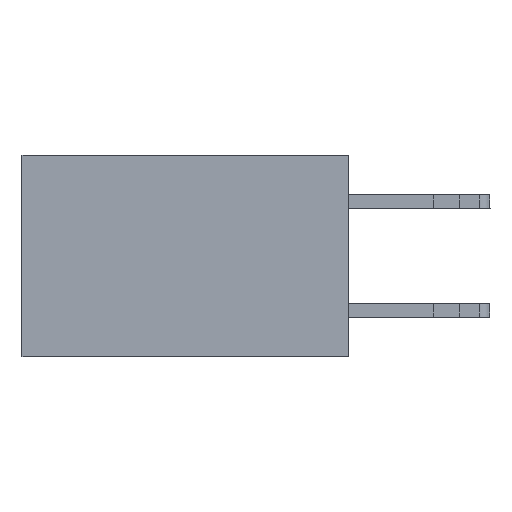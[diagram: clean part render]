
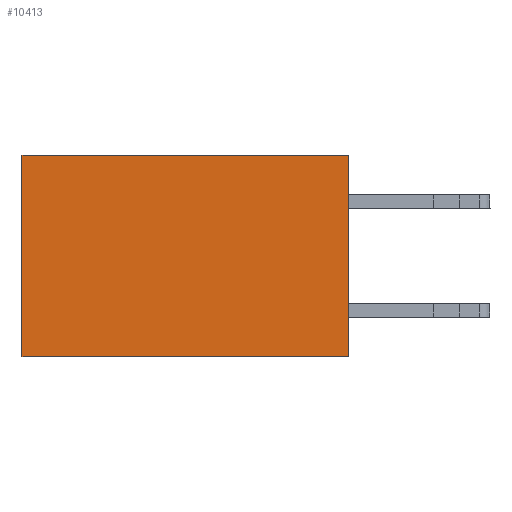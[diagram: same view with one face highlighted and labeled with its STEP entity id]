
A CAD part, left-side view. The second image highlights one B-rep face of the part: STEP entity #10413.
In plain terms, the highlighted planar face has unit normal (-1, 0, 0).
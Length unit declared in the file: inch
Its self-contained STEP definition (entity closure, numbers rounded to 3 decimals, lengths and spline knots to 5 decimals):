
#1106 = CARTESIAN_POINT ( 'NONE',  ( 0.2615, 0., -0.37 ) ) ;
#1721 = EDGE_CURVE ( 'NONE', #8797, #2682, #7178, .T. ) ;
#1941 = DIRECTION ( 'NONE',  ( 0., 0., -1. ) ) ;
#2469 = VECTOR ( 'NONE', #15292, 39.37008 ) ;
#2682 = VERTEX_POINT ( 'NONE', #7598 ) ;
#3089 = EDGE_CURVE ( 'NONE', #3127, #8797, #10516, .T. ) ;
#3127 = VERTEX_POINT ( 'NONE', #13555 ) ;
#3202 = ORIENTED_EDGE ( 'NONE', *, *, #16057, .T. ) ;
#3673 = DIRECTION ( 'NONE',  ( 1., 0., 0. ) ) ;
#4519 = AXIS2_PLACEMENT_3D ( 'NONE', #15950, #3673, #1941 ) ;
#4610 = ORIENTED_EDGE ( 'NONE', *, *, #1721, .F. ) ;
#5756 = DIRECTION ( 'NONE',  ( 0., 1., 0. ) ) ;
#5935 = CARTESIAN_POINT ( 'NONE',  ( 0.2615, 0.6, 0. ) ) ;
#7178 = LINE ( 'NONE', #11849, #13612 ) ;
#7293 = LINE ( 'NONE', #16848, #8883 ) ;
#7337 = DIRECTION ( 'NONE',  ( 0., 0., -1. ) ) ;
#7400 = ORIENTED_EDGE ( 'NONE', *, *, #3089, .F. ) ;
#7489 = DIRECTION ( 'NONE',  ( 0., 1., 0. ) ) ;
#7598 = CARTESIAN_POINT ( 'NONE',  ( 0.2615, 0.6, -0.37 ) ) ;
#7959 = EDGE_CURVE ( 'NONE', #9068, #2682, #10483, .T. ) ;
#8302 = ORIENTED_EDGE ( 'NONE', *, *, #7959, .T. ) ;
#8429 = PLANE ( 'NONE',  #4519 ) ;
#8797 = VERTEX_POINT ( 'NONE', #19574 ) ;
#8883 = VECTOR ( 'NONE', #7489, 39.37008 ) ;
#9068 = VERTEX_POINT ( 'NONE', #5935 ) ;
#10413 = ADVANCED_FACE ( 'NONE', ( #12794 ), #8429, .F. ) ;
#10483 = LINE ( 'NONE', #16701, #17143 ) ;
#10516 = LINE ( 'NONE', #1106, #2469 ) ;
#11034 = EDGE_LOOP ( 'NONE', ( #8302, #4610, #7400, #3202 ) ) ;
#11849 = CARTESIAN_POINT ( 'NONE',  ( 0.2615, 0., -0.37 ) ) ;
#12794 = FACE_OUTER_BOUND ( 'NONE', #11034, .T. ) ;
#13555 = CARTESIAN_POINT ( 'NONE',  ( 0.2615, 0., 0. ) ) ;
#13612 = VECTOR ( 'NONE', #5756, 39.37008 ) ;
#15292 = DIRECTION ( 'NONE',  ( 0., 0., -1. ) ) ;
#15950 = CARTESIAN_POINT ( 'NONE',  ( 0.2615, 0., -0.37 ) ) ;
#16057 = EDGE_CURVE ( 'NONE', #3127, #9068, #7293, .T. ) ;
#16701 = CARTESIAN_POINT ( 'NONE',  ( 0.2615, 0.6, -0.37 ) ) ;
#16848 = CARTESIAN_POINT ( 'NONE',  ( 0.2615, 0., 0. ) ) ;
#17143 = VECTOR ( 'NONE', #7337, 39.37008 ) ;
#19574 = CARTESIAN_POINT ( 'NONE',  ( 0.2615, 0., -0.37 ) ) ;
